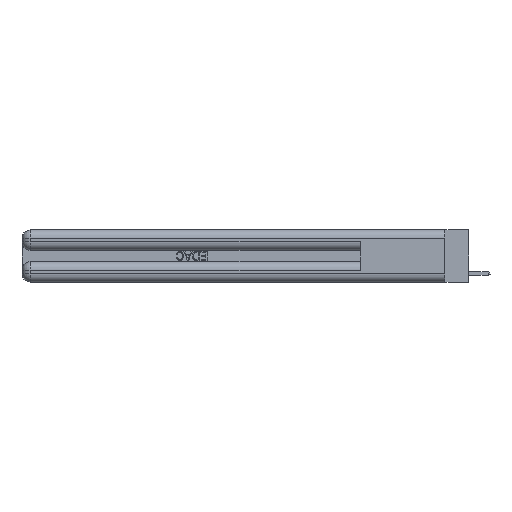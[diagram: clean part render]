
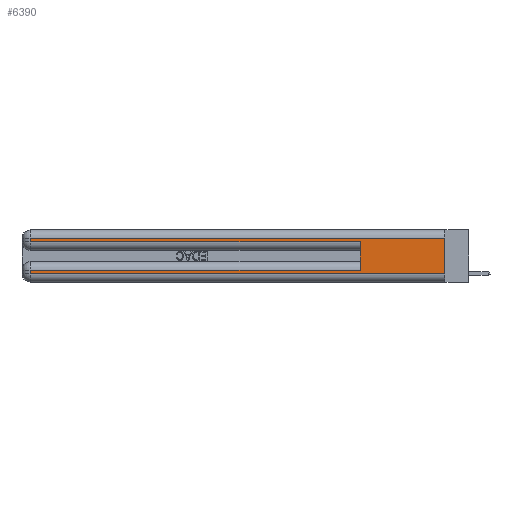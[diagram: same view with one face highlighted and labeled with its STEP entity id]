
A CAD part, left-side view. The second image highlights one B-rep face of the part: STEP entity #6390.
In plain terms, the highlighted planar face has unit normal (-1, 0, 0).
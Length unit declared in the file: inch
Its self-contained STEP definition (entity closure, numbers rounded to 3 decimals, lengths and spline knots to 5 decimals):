
#793 = PLANE ( 'NONE',  #24028 ) ;
#848 = EDGE_CURVE ( 'NONE', #14681, #10362, #28169, .T. ) ;
#898 = DIRECTION ( 'NONE',  ( 0., 1., 0. ) ) ;
#1862 = VERTEX_POINT ( 'NONE', #29541 ) ;
#2099 = CARTESIAN_POINT ( 'NONE',  ( 0., 2.94, 0.37 ) ) ;
#2390 = DIRECTION ( 'NONE',  ( 0., 0., -1. ) ) ;
#2516 = VECTOR ( 'NONE', #26722, 39.37008 ) ;
#2539 = VERTEX_POINT ( 'NONE', #9693 ) ;
#3067 = FACE_OUTER_BOUND ( 'NONE', #12577, .T. ) ;
#3742 = ORIENTED_EDGE ( 'NONE', *, *, #24762, .T. ) ;
#6390 = ADVANCED_FACE ( 'NONE', ( #3067 ), #793, .F. ) ;
#6767 = CARTESIAN_POINT ( 'NONE',  ( 0., 0.6, 0.285 ) ) ;
#7570 = LINE ( 'NONE', #9991, #9064 ) ;
#9064 = VECTOR ( 'NONE', #898, 39.37008 ) ;
#9130 = VERTEX_POINT ( 'NONE', #26880 ) ;
#9644 = CARTESIAN_POINT ( 'NONE',  ( 0., 0., 0.285 ) ) ;
#9693 = CARTESIAN_POINT ( 'NONE',  ( 0., 0., 0.06 ) ) ;
#9730 = ORIENTED_EDGE ( 'NONE', *, *, #20125, .T. ) ;
#9991 = CARTESIAN_POINT ( 'NONE',  ( 0., 0., 0.31 ) ) ;
#10362 = VERTEX_POINT ( 'NONE', #6767 ) ;
#11276 = EDGE_CURVE ( 'NONE', #29368, #2539, #21043, .T. ) ;
#11740 = VECTOR ( 'NONE', #12278, 39.37008 ) ;
#12204 = DIRECTION ( 'NONE',  ( 0., -1., 0. ) ) ;
#12278 = DIRECTION ( 'NONE',  ( 0., 0., 1. ) ) ;
#12576 = ORIENTED_EDGE ( 'NONE', *, *, #27341, .T. ) ;
#12577 = EDGE_LOOP ( 'NONE', ( #26183, #9730, #12576, #3742, #19509, #25421, #23948, #14236 ) ) ;
#12692 = EDGE_CURVE ( 'NONE', #17781, #21368, #22812, .T. ) ;
#13055 = CARTESIAN_POINT ( 'NONE',  ( 0., 0., 0.085 ) ) ;
#14236 = ORIENTED_EDGE ( 'NONE', *, *, #22468, .T. ) ;
#14681 = VERTEX_POINT ( 'NONE', #20314 ) ;
#15524 = VECTOR ( 'NONE', #27715, 39.37008 ) ;
#15790 = CARTESIAN_POINT ( 'NONE',  ( 0., 2.94, 0.37 ) ) ;
#16499 = CARTESIAN_POINT ( 'NONE',  ( 0., 0.6, 0.145 ) ) ;
#17249 = DIRECTION ( 'NONE',  ( 0., 0., -1. ) ) ;
#17470 = LINE ( 'NONE', #15790, #2516 ) ;
#17781 = VERTEX_POINT ( 'NONE', #20791 ) ;
#18939 = DIRECTION ( 'NONE',  ( 1., 0., 0. ) ) ;
#19276 = LINE ( 'NONE', #9644, #28084 ) ;
#19509 = ORIENTED_EDGE ( 'NONE', *, *, #848, .F. ) ;
#19769 = CARTESIAN_POINT ( 'NONE',  ( 0., 0., 0.31 ) ) ;
#20001 = LINE ( 'NONE', #13055, #26639 ) ;
#20125 = EDGE_CURVE ( 'NONE', #29368, #1862, #7570, .T. ) ;
#20314 = CARTESIAN_POINT ( 'NONE',  ( 0., 0.6, 0.085 ) ) ;
#20791 = CARTESIAN_POINT ( 'NONE',  ( 0., 2.94, 0.085 ) ) ;
#21043 = LINE ( 'NONE', #27860, #15524 ) ;
#21368 = VERTEX_POINT ( 'NONE', #25323 ) ;
#21830 = DIRECTION ( 'NONE',  ( 0., 1., 0. ) ) ;
#22468 = EDGE_CURVE ( 'NONE', #21368, #2539, #24440, .T. ) ;
#22766 = VECTOR ( 'NONE', #2390, 39.37008 ) ;
#22812 = LINE ( 'NONE', #2099, #22766 ) ;
#23158 = VECTOR ( 'NONE', #24583, 39.37008 ) ;
#23948 = ORIENTED_EDGE ( 'NONE', *, *, #12692, .T. ) ;
#24028 = AXIS2_PLACEMENT_3D ( 'NONE', #28781, #18939, #17249 ) ;
#24440 = LINE ( 'NONE', #29405, #23158 ) ;
#24583 = DIRECTION ( 'NONE',  ( 0., -1., 0. ) ) ;
#24762 = EDGE_CURVE ( 'NONE', #9130, #10362, #19276, .T. ) ;
#25323 = CARTESIAN_POINT ( 'NONE',  ( 0., 2.94, 0.06 ) ) ;
#25421 = ORIENTED_EDGE ( 'NONE', *, *, #26436, .T. ) ;
#26183 = ORIENTED_EDGE ( 'NONE', *, *, #11276, .F. ) ;
#26436 = EDGE_CURVE ( 'NONE', #14681, #17781, #20001, .T. ) ;
#26639 = VECTOR ( 'NONE', #21830, 39.37008 ) ;
#26722 = DIRECTION ( 'NONE',  ( 0., 0., -1. ) ) ;
#26880 = CARTESIAN_POINT ( 'NONE',  ( 0., 2.94, 0.285 ) ) ;
#27341 = EDGE_CURVE ( 'NONE', #1862, #9130, #17470, .T. ) ;
#27715 = DIRECTION ( 'NONE',  ( 0., 0., -1. ) ) ;
#27860 = CARTESIAN_POINT ( 'NONE',  ( 0., 0., 0.37 ) ) ;
#28084 = VECTOR ( 'NONE', #12204, 39.37008 ) ;
#28169 = LINE ( 'NONE', #16499, #11740 ) ;
#28781 = CARTESIAN_POINT ( 'NONE',  ( 0., 0., 0.37 ) ) ;
#29368 = VERTEX_POINT ( 'NONE', #19769 ) ;
#29405 = CARTESIAN_POINT ( 'NONE',  ( 0., 0., 0.06 ) ) ;
#29541 = CARTESIAN_POINT ( 'NONE',  ( 0., 2.94, 0.31 ) ) ;
